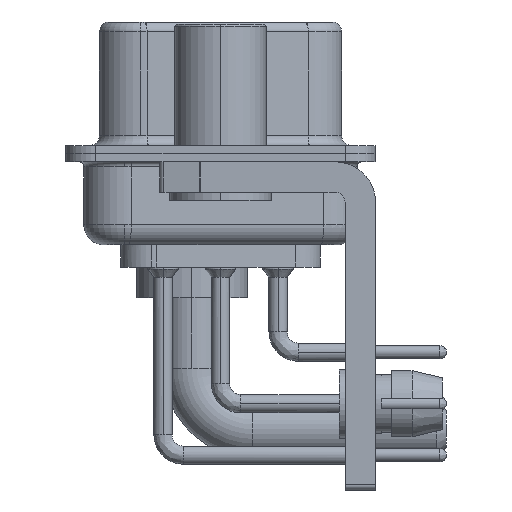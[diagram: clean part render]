
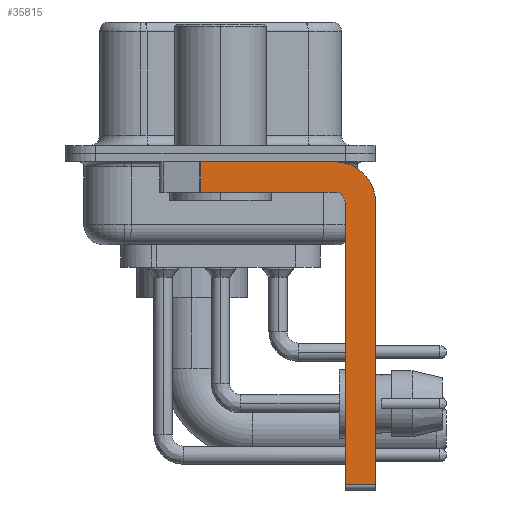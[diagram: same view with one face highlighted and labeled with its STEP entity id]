
A CAD part, left-side view. The second image highlights one B-rep face of the part: STEP entity #35815.
In plain terms, the highlighted planar face has unit normal (-1, 0, 0).
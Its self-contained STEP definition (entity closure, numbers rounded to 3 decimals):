
#1080 = FACE_OUTER_BOUND ( 'NONE', #4523, .T. ) ;
#2287 = ORIENTED_EDGE ( 'NONE', *, *, #21374, .T. ) ;
#2660 = ORIENTED_EDGE ( 'NONE', *, *, #16541, .F. ) ;
#2665 = CARTESIAN_POINT ( 'NONE',  ( -2.9, -7.65, -2.4 ) ) ;
#3001 = VERTEX_POINT ( 'NONE', #37976 ) ;
#4242 = CARTESIAN_POINT ( 'NONE',  ( -2.9, 0.978, -0.4 ) ) ;
#4523 = EDGE_LOOP ( 'NONE', ( #2660, #35555, #34676, #37112, #11948, #2287, #8606, #6924 ) ) ;
#4813 = EDGE_CURVE ( 'NONE', #15468, #16586, #13756, .T. ) ;
#5487 = EDGE_CURVE ( 'NONE', #22431, #3001, #5842, .T. ) ;
#5625 = LINE ( 'NONE', #24453, #27698 ) ;
#5842 = LINE ( 'NONE', #28575, #9885 ) ;
#5908 = LINE ( 'NONE', #18423, #21864 ) ;
#6188 = LINE ( 'NONE', #12538, #35873 ) ;
#6256 = VERTEX_POINT ( 'NONE', #2665 ) ;
#6924 = ORIENTED_EDGE ( 'NONE', *, *, #31758, .F. ) ;
#7607 = CARTESIAN_POINT ( 'NONE',  ( -2.9, -5.65, -2.4 ) ) ;
#7618 = DIRECTION ( 'NONE',  ( 0., 0., -1. ) ) ;
#7819 = AXIS2_PLACEMENT_3D ( 'NONE', #38622, #38825, #35953 ) ;
#8606 = ORIENTED_EDGE ( 'NONE', *, *, #29662, .F. ) ;
#9885 = VECTOR ( 'NONE', #27953, 1000. ) ;
#9928 = EDGE_CURVE ( 'NONE', #16586, #3001, #5908, .T. ) ;
#10660 = DIRECTION ( 'NONE',  ( 0., 0., 1. ) ) ;
#11398 = CARTESIAN_POINT ( 'NONE',  ( -2.9, -6.15, -16.35 ) ) ;
#11948 = ORIENTED_EDGE ( 'NONE', *, *, #15542, .F. ) ;
#12538 = CARTESIAN_POINT ( 'NONE',  ( -2.9, -6.15, -16.6 ) ) ;
#12684 = VERTEX_POINT ( 'NONE', #11398 ) ;
#13656 = CARTESIAN_POINT ( 'NONE',  ( -2.9, -6.15, -2.4 ) ) ;
#13756 = CIRCLE ( 'NONE', #36603, 0.5 ) ;
#14032 = CARTESIAN_POINT ( 'NONE',  ( -2.9, -7.65, -16.35 ) ) ;
#15468 = VERTEX_POINT ( 'NONE', #13656 ) ;
#15542 = EDGE_CURVE ( 'NONE', #12684, #15468, #6188, .T. ) ;
#16541 = EDGE_CURVE ( 'NONE', #22431, #36738, #19216, .T. ) ;
#16586 = VERTEX_POINT ( 'NONE', #31692 ) ;
#18423 = CARTESIAN_POINT ( 'NONE',  ( -2.9, -5.65, -1.9 ) ) ;
#19216 = LINE ( 'NONE', #25735, #22252 ) ;
#21374 = EDGE_CURVE ( 'NONE', #12684, #35384, #5625, .T. ) ;
#21864 = VECTOR ( 'NONE', #30896, 1000. ) ;
#22252 = VECTOR ( 'NONE', #29228, 1000. ) ;
#22431 = VERTEX_POINT ( 'NONE', #4242 ) ;
#23391 = DIRECTION ( 'NONE',  ( 1., 0., 0. ) ) ;
#23589 = CARTESIAN_POINT ( 'NONE',  ( -2.9, -5.65, -2.4 ) ) ;
#24453 = CARTESIAN_POINT ( 'NONE',  ( -2.9, -5.65, -16.35 ) ) ;
#24604 = CARTESIAN_POINT ( 'NONE',  ( -2.9, -5.65, -0.4 ) ) ;
#25735 = CARTESIAN_POINT ( 'NONE',  ( -2.9, 3., -0.4 ) ) ;
#27076 = DIRECTION ( 'NONE',  ( 0., 0., -1. ) ) ;
#27698 = VECTOR ( 'NONE', #36705, 1000. ) ;
#27953 = DIRECTION ( 'NONE',  ( 0., 0., -1. ) ) ;
#28575 = CARTESIAN_POINT ( 'NONE',  ( -2.9, 0.978, -1.9 ) ) ;
#29228 = DIRECTION ( 'NONE',  ( 0., -1., 0. ) ) ;
#29662 = EDGE_CURVE ( 'NONE', #6256, #35384, #40298, .T. ) ;
#29934 = PLANE ( 'NONE',  #35505 ) ;
#30896 = DIRECTION ( 'NONE',  ( 0., 1., 0. ) ) ;
#31438 = CIRCLE ( 'NONE', #7819, 2. ) ;
#31585 = DIRECTION ( 'NONE',  ( 0., 0., 1. ) ) ;
#31692 = CARTESIAN_POINT ( 'NONE',  ( -2.9, -5.65, -1.9 ) ) ;
#31758 = EDGE_CURVE ( 'NONE', #36738, #6256, #31438, .T. ) ;
#34676 = ORIENTED_EDGE ( 'NONE', *, *, #9928, .F. ) ;
#35384 = VERTEX_POINT ( 'NONE', #14032 ) ;
#35505 = AXIS2_PLACEMENT_3D ( 'NONE', #23589, #23391, #7618 ) ;
#35555 = ORIENTED_EDGE ( 'NONE', *, *, #5487, .T. ) ;
#35815 = ADVANCED_FACE ( 'NONE', ( #1080 ), #29934, .F. ) ;
#35873 = VECTOR ( 'NONE', #31585, 1000. ) ;
#35953 = DIRECTION ( 'NONE',  ( 0., 0., -1. ) ) ;
#36245 = CARTESIAN_POINT ( 'NONE',  ( -2.9, -7.65, -2.4 ) ) ;
#36603 = AXIS2_PLACEMENT_3D ( 'NONE', #7607, #38685, #10660 ) ;
#36705 = DIRECTION ( 'NONE',  ( 0., -1., 0. ) ) ;
#36738 = VERTEX_POINT ( 'NONE', #24604 ) ;
#37112 = ORIENTED_EDGE ( 'NONE', *, *, #4813, .F. ) ;
#37802 = VECTOR ( 'NONE', #27076, 1000. ) ;
#37976 = CARTESIAN_POINT ( 'NONE',  ( -2.9, 0.978, -1.9 ) ) ;
#38622 = CARTESIAN_POINT ( 'NONE',  ( -2.9, -5.65, -2.4 ) ) ;
#38685 = DIRECTION ( 'NONE',  ( -1., 0., 0. ) ) ;
#38825 = DIRECTION ( 'NONE',  ( 1., 0., 0. ) ) ;
#40298 = LINE ( 'NONE', #36245, #37802 ) ;
